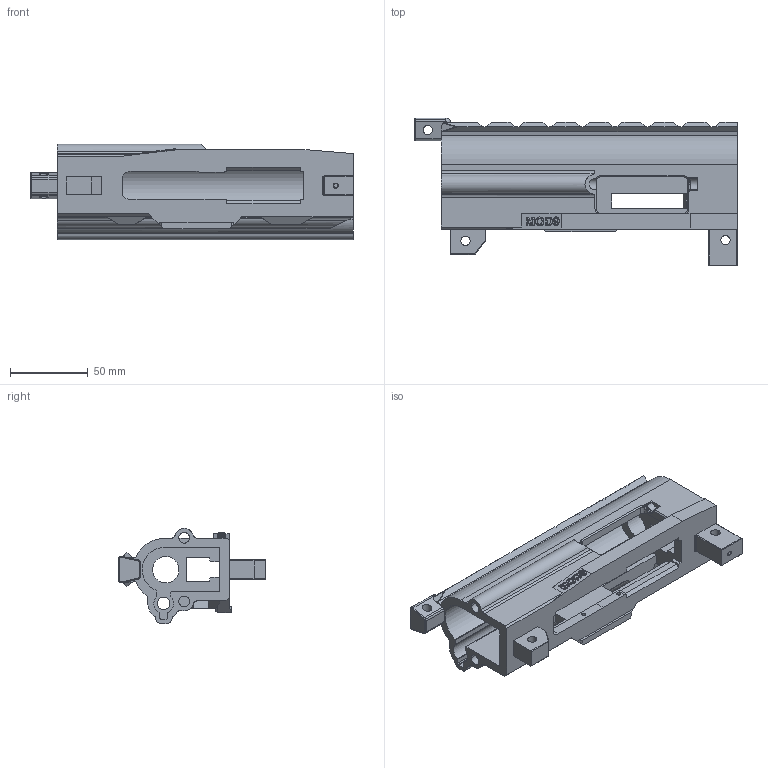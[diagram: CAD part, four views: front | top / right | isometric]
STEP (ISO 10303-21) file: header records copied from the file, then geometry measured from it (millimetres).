
FILE_DESCRIPTION(('STEP AP214'),'1');
FILE_NAME('Mod9 Upper Receiver Final.stp','2020-09-28T22:42:26',(' '),(' '),'Spatial InterOp 3D',' ',' ');
FILE_SCHEMA(('AUTOMOTIVE_DESIGN { 1 0 10303 214 1 1 1 1 }'));
Length unit declared in the file: metre
Products named in the file (1): Solid
Bounding box: 207.36 x 94.9 x 61.22 mm (x, y, z)
Volume: 250557.7 mm3; surface area: 90176.2 mm2
Topology: 1 solids, 1 shells, 555 faces, 1572 edges, 1025 vertices
Faces by surface type: plane 235, cylinder 168, bspline 110, cone 23, torus 19
Entity records: 20368 total; most frequent: CARTESIAN_POINT 6535, ORIENTED_EDGE 3144, DIRECTION 2509, EDGE_CURVE 1572, VERTEX_POINT 1025, LINE 891, VECTOR 891, AXIS2_PLACEMENT_3D 809
